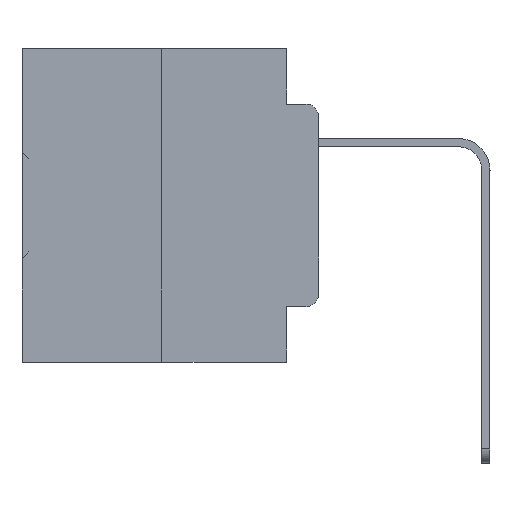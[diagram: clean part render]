
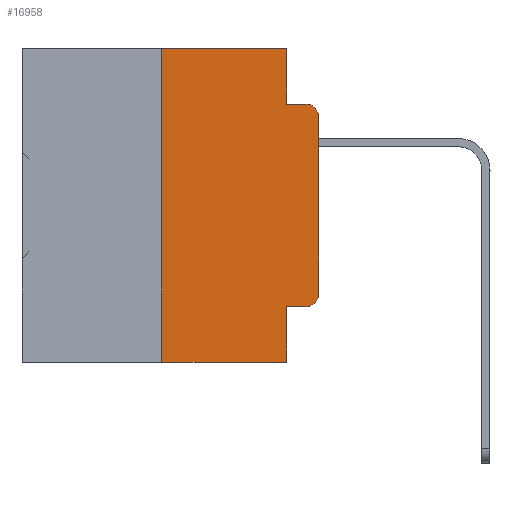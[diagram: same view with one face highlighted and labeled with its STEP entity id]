
A CAD part, left-side view. The second image highlights one B-rep face of the part: STEP entity #16958.
In plain terms, the highlighted planar face has unit normal (-1, 0, 0).
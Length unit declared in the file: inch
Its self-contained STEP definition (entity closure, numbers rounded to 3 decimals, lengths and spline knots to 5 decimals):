
#430 = VERTEX_POINT ( 'NONE', #29102 ) ;
#512 = CARTESIAN_POINT ( 'NONE',  ( 0., 0.051, -0.4115 ) ) ;
#823 = CARTESIAN_POINT ( 'NONE',  ( 0., 0.473, 0. ) ) ;
#1599 = VERTEX_POINT ( 'NONE', #6839 ) ;
#1712 = LINE ( 'NONE', #823, #22310 ) ;
#1879 = CARTESIAN_POINT ( 'NONE',  ( 0., 0.25, 0. ) ) ;
#3043 = VECTOR ( 'NONE', #16529, 39.37008 ) ;
#3618 = VERTEX_POINT ( 'NONE', #512 ) ;
#3763 = DIRECTION ( 'NONE',  ( 0., -1., 0. ) ) ;
#4006 = VERTEX_POINT ( 'NONE', #28503 ) ;
#4007 = CARTESIAN_POINT ( 'NONE',  ( 0., 0.051, 0. ) ) ;
#5482 = EDGE_CURVE ( 'NONE', #1599, #13539, #9663, .T. ) ;
#5925 = CARTESIAN_POINT ( 'NONE',  ( 0., 0.051, -0.0885 ) ) ;
#6839 = CARTESIAN_POINT ( 'NONE',  ( 0., 0.25, -0.5 ) ) ;
#7147 = VECTOR ( 'NONE', #33312, 39.37008 ) ;
#7503 = PLANE ( 'NONE',  #12579 ) ;
#7536 = CARTESIAN_POINT ( 'NONE',  ( 0., 0.051, 0. ) ) ;
#7638 = ORIENTED_EDGE ( 'NONE', *, *, #16656, .T. ) ;
#7763 = ORIENTED_EDGE ( 'NONE', *, *, #5482, .F. ) ;
#7906 = CARTESIAN_POINT ( 'NONE',  ( 0., 0.02, -0.1085 ) ) ;
#8521 = FACE_OUTER_BOUND ( 'NONE', #37523, .T. ) ;
#8953 = CIRCLE ( 'NONE', #26261, 0.02 ) ;
#9246 = ORIENTED_EDGE ( 'NONE', *, *, #19042, .T. ) ;
#9663 = LINE ( 'NONE', #21657, #27010 ) ;
#9823 = CARTESIAN_POINT ( 'NONE',  ( 0., 0.051, -0.4115 ) ) ;
#9882 = CARTESIAN_POINT ( 'NONE',  ( 0., 0., -0.1085 ) ) ;
#10636 = DIRECTION ( 'NONE',  ( 1., 0., 0. ) ) ;
#10727 = LINE ( 'NONE', #18615, #17123 ) ;
#10824 = LINE ( 'NONE', #7536, #3043 ) ;
#11041 = CARTESIAN_POINT ( 'NONE',  ( 0., 0.051, 0. ) ) ;
#12070 = EDGE_CURVE ( 'NONE', #13539, #20561, #1712, .T. ) ;
#12165 = ORIENTED_EDGE ( 'NONE', *, *, #26684, .T. ) ;
#12579 = AXIS2_PLACEMENT_3D ( 'NONE', #37114, #10636, #19549 ) ;
#13539 = VERTEX_POINT ( 'NONE', #1879 ) ;
#13693 = DIRECTION ( 'NONE',  ( 0., 0., -1. ) ) ;
#15361 = DIRECTION ( 'NONE',  ( 0., 0., 1. ) ) ;
#16211 = ORIENTED_EDGE ( 'NONE', *, *, #12070, .F. ) ;
#16529 = DIRECTION ( 'NONE',  ( 0., 0., -1. ) ) ;
#16656 = EDGE_CURVE ( 'NONE', #33616, #29883, #36023, .T. ) ;
#16958 = ADVANCED_FACE ( 'NONE', ( #8521 ), #7503, .F. ) ;
#17123 = VECTOR ( 'NONE', #3763, 39.37008 ) ;
#18356 = DIRECTION ( 'NONE',  ( 0., 0., 1. ) ) ;
#18615 = CARTESIAN_POINT ( 'NONE',  ( 0., 0.473, -0.5 ) ) ;
#18797 = DIRECTION ( 'NONE',  ( -1., 0., 0. ) ) ;
#18801 = ORIENTED_EDGE ( 'NONE', *, *, #29529, .F. ) ;
#19042 = EDGE_CURVE ( 'NONE', #430, #33616, #36810, .T. ) ;
#19549 = DIRECTION ( 'NONE',  ( 0., 0., -1. ) ) ;
#19691 = VERTEX_POINT ( 'NONE', #27809 ) ;
#20180 = LINE ( 'NONE', #9823, #35309 ) ;
#20561 = VERTEX_POINT ( 'NONE', #11041 ) ;
#21523 = EDGE_CURVE ( 'NONE', #28076, #4006, #30615, .T. ) ;
#21657 = CARTESIAN_POINT ( 'NONE',  ( 0., 0.25, 0. ) ) ;
#22310 = VECTOR ( 'NONE', #24235, 39.37008 ) ;
#22446 = ORIENTED_EDGE ( 'NONE', *, *, #21523, .F. ) ;
#22938 = ORIENTED_EDGE ( 'NONE', *, *, #30031, .T. ) ;
#23592 = DIRECTION ( 'NONE',  ( 0., -1., 0. ) ) ;
#23757 = VECTOR ( 'NONE', #23592, 39.37008 ) ;
#24235 = DIRECTION ( 'NONE',  ( 0., -1., 0. ) ) ;
#26261 = AXIS2_PLACEMENT_3D ( 'NONE', #7906, #33898, #13693 ) ;
#26359 = VECTOR ( 'NONE', #15361, 39.37008 ) ;
#26684 = EDGE_CURVE ( 'NONE', #3618, #430, #20180, .T. ) ;
#27010 = VECTOR ( 'NONE', #18356, 39.37008 ) ;
#27809 = CARTESIAN_POINT ( 'NONE',  ( 0., 0.051, -0.5 ) ) ;
#28076 = VERTEX_POINT ( 'NONE', #29577 ) ;
#28503 = CARTESIAN_POINT ( 'NONE',  ( 0., 0.02, -0.0885 ) ) ;
#29102 = CARTESIAN_POINT ( 'NONE',  ( 0., 0.02, -0.4115 ) ) ;
#29529 = EDGE_CURVE ( 'NONE', #3618, #19691, #36941, .T. ) ;
#29577 = CARTESIAN_POINT ( 'NONE',  ( 0., 0.051, -0.0885 ) ) ;
#29874 = DIRECTION ( 'NONE',  ( 0., -1., 0. ) ) ;
#29883 = VERTEX_POINT ( 'NONE', #9882 ) ;
#30031 = EDGE_CURVE ( 'NONE', #29883, #4006, #8953, .T. ) ;
#30050 = CARTESIAN_POINT ( 'NONE',  ( 0., 0., 0. ) ) ;
#30615 = LINE ( 'NONE', #5925, #23757 ) ;
#30983 = EDGE_CURVE ( 'NONE', #1599, #19691, #10727, .T. ) ;
#32275 = CARTESIAN_POINT ( 'NONE',  ( 0., 0., -0.3915 ) ) ;
#33312 = DIRECTION ( 'NONE',  ( 0., 0., -1. ) ) ;
#33616 = VERTEX_POINT ( 'NONE', #32275 ) ;
#33898 = DIRECTION ( 'NONE',  ( -1., 0., 0. ) ) ;
#34194 = EDGE_CURVE ( 'NONE', #20561, #28076, #10824, .T. ) ;
#34392 = AXIS2_PLACEMENT_3D ( 'NONE', #36332, #18797, #36723 ) ;
#35309 = VECTOR ( 'NONE', #29874, 39.37008 ) ;
#36023 = LINE ( 'NONE', #30050, #26359 ) ;
#36332 = CARTESIAN_POINT ( 'NONE',  ( 0., 0.02, -0.3915 ) ) ;
#36632 = ORIENTED_EDGE ( 'NONE', *, *, #30983, .T. ) ;
#36723 = DIRECTION ( 'NONE',  ( 0., 0., -1. ) ) ;
#36810 = CIRCLE ( 'NONE', #34392, 0.02 ) ;
#36941 = LINE ( 'NONE', #4007, #7147 ) ;
#37114 = CARTESIAN_POINT ( 'NONE',  ( 0., 0.473, 0. ) ) ;
#37523 = EDGE_LOOP ( 'NONE', ( #7638, #22938, #22446, #37991, #16211, #7763, #36632, #18801, #12165, #9246 ) ) ;
#37991 = ORIENTED_EDGE ( 'NONE', *, *, #34194, .F. ) ;
